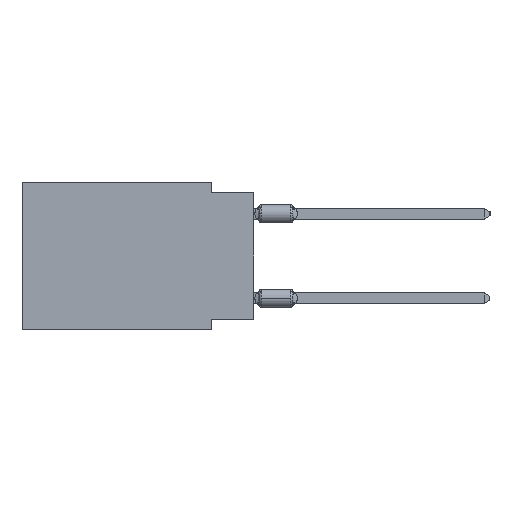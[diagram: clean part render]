
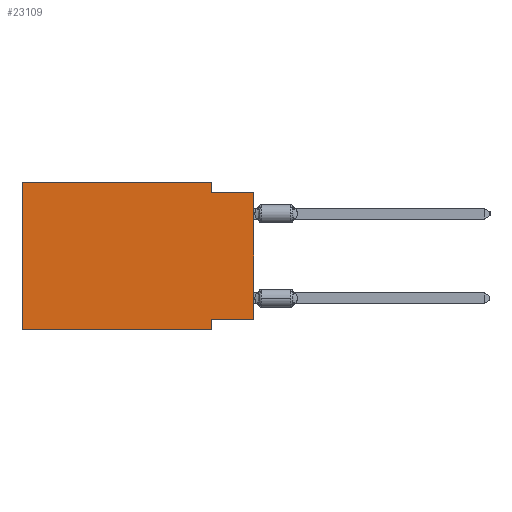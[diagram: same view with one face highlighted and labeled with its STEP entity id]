
A CAD part, left-side view. The second image highlights one B-rep face of the part: STEP entity #23109.
In plain terms, the highlighted planar face has unit normal (-1, 0, 0).
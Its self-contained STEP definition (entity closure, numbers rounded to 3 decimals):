
#933 = DIRECTION ( 'NONE',  ( 0., 1., 0. ) ) ;
#1464 = CARTESIAN_POINT ( 'NONE',  ( 0., 0., -8.255 ) ) ;
#4327 = VECTOR ( 'NONE', #4567, 1000. ) ;
#4567 = DIRECTION ( 'NONE',  ( 0., 0., -1. ) ) ;
#4967 = CARTESIAN_POINT ( 'NONE',  ( 0., 0., 0. ) ) ;
#5822 = ORIENTED_EDGE ( 'NONE', *, *, #59109, .F. ) ;
#6169 = FACE_OUTER_BOUND ( 'NONE', #55028, .T. ) ;
#6248 = CARTESIAN_POINT ( 'NONE',  ( 0., 13.97, 0. ) ) ;
#6306 = CARTESIAN_POINT ( 'NONE',  ( 0., 0., -8.255 ) ) ;
#6404 = EDGE_CURVE ( 'NONE', #53952, #66199, #46288, .T. ) ;
#6507 = PLANE ( 'NONE',  #38197 ) ;
#9650 = VECTOR ( 'NONE', #70091, 1000. ) ;
#11350 = LINE ( 'NONE', #65529, #69585 ) ;
#12468 = LINE ( 'NONE', #50595, #31604 ) ;
#14193 = ORIENTED_EDGE ( 'NONE', *, *, #14325, .T. ) ;
#14324 = EDGE_CURVE ( 'NONE', #34864, #66199, #17049, .T. ) ;
#14325 = EDGE_CURVE ( 'NONE', #20962, #28728, #11350, .T. ) ;
#17049 = LINE ( 'NONE', #4967, #24068 ) ;
#20962 = VERTEX_POINT ( 'NONE', #66958 ) ;
#22067 = DIRECTION ( 'NONE',  ( 0., 0., 1. ) ) ;
#22688 = CARTESIAN_POINT ( 'NONE',  ( 0., 2.54, -8.89 ) ) ;
#22704 = LINE ( 'NONE', #6306, #68304 ) ;
#23109 = ADVANCED_FACE ( 'NONE', ( #6169 ), #6507, .F. ) ;
#24068 = VECTOR ( 'NONE', #22067, 1000. ) ;
#25705 = EDGE_CURVE ( 'NONE', #61321, #30033, #12468, .T. ) ;
#26037 = CARTESIAN_POINT ( 'NONE',  ( 0., 2.54, -0.635 ) ) ;
#26087 = EDGE_CURVE ( 'NONE', #50773, #28728, #60484, .T. ) ;
#27874 = EDGE_CURVE ( 'NONE', #34864, #50773, #22704, .T. ) ;
#28728 = VERTEX_POINT ( 'NONE', #22688 ) ;
#29919 = CARTESIAN_POINT ( 'NONE',  ( 0., 0., -0.635 ) ) ;
#30033 = VERTEX_POINT ( 'NONE', #44791 ) ;
#30485 = EDGE_CURVE ( 'NONE', #30033, #53952, #37331, .T. ) ;
#31604 = VECTOR ( 'NONE', #60921, 1000. ) ;
#32894 = DIRECTION ( 'NONE',  ( 0., 0., -1. ) ) ;
#33108 = DIRECTION ( 'NONE',  ( 0., -1., 0. ) ) ;
#34864 = VERTEX_POINT ( 'NONE', #1464 ) ;
#37331 = LINE ( 'NONE', #59735, #9650 ) ;
#38197 = AXIS2_PLACEMENT_3D ( 'NONE', #44278, #49270, #32894 ) ;
#40005 = VECTOR ( 'NONE', #66470, 1000. ) ;
#44278 = CARTESIAN_POINT ( 'NONE',  ( 0., 13.97, 0. ) ) ;
#44791 = CARTESIAN_POINT ( 'NONE',  ( 0., 2.54, 0. ) ) ;
#46288 = LINE ( 'NONE', #29919, #47974 ) ;
#47299 = ORIENTED_EDGE ( 'NONE', *, *, #25705, .F. ) ;
#47974 = VECTOR ( 'NONE', #51631, 1000. ) ;
#48931 = ORIENTED_EDGE ( 'NONE', *, *, #30485, .F. ) ;
#49270 = DIRECTION ( 'NONE',  ( 1., 0., 0. ) ) ;
#49350 = LINE ( 'NONE', #6248, #40005 ) ;
#49409 = CARTESIAN_POINT ( 'NONE',  ( 0., 13.97, 0. ) ) ;
#50046 = ORIENTED_EDGE ( 'NONE', *, *, #14324, .T. ) ;
#50595 = CARTESIAN_POINT ( 'NONE',  ( 0., 13.97, 0. ) ) ;
#50773 = VERTEX_POINT ( 'NONE', #61368 ) ;
#51324 = ORIENTED_EDGE ( 'NONE', *, *, #6404, .F. ) ;
#51631 = DIRECTION ( 'NONE',  ( 0., -1., 0. ) ) ;
#53370 = CARTESIAN_POINT ( 'NONE',  ( 0., 2.54, -8.89 ) ) ;
#53952 = VERTEX_POINT ( 'NONE', #26037 ) ;
#55028 = EDGE_LOOP ( 'NONE', ( #50046, #51324, #48931, #47299, #5822, #14193, #58346, #61771 ) ) ;
#58346 = ORIENTED_EDGE ( 'NONE', *, *, #26087, .F. ) ;
#59109 = EDGE_CURVE ( 'NONE', #20962, #61321, #49350, .T. ) ;
#59735 = CARTESIAN_POINT ( 'NONE',  ( 0., 2.54, 0. ) ) ;
#60484 = LINE ( 'NONE', #53370, #4327 ) ;
#60921 = DIRECTION ( 'NONE',  ( 0., -1., 0. ) ) ;
#61321 = VERTEX_POINT ( 'NONE', #49409 ) ;
#61368 = CARTESIAN_POINT ( 'NONE',  ( 0., 2.54, -8.255 ) ) ;
#61771 = ORIENTED_EDGE ( 'NONE', *, *, #27874, .F. ) ;
#65529 = CARTESIAN_POINT ( 'NONE',  ( 0., 13.97, -8.89 ) ) ;
#66199 = VERTEX_POINT ( 'NONE', #66884 ) ;
#66470 = DIRECTION ( 'NONE',  ( 0., 0., 1. ) ) ;
#66884 = CARTESIAN_POINT ( 'NONE',  ( 0., 0., -0.635 ) ) ;
#66958 = CARTESIAN_POINT ( 'NONE',  ( 0., 13.97, -8.89 ) ) ;
#68304 = VECTOR ( 'NONE', #933, 1000. ) ;
#69585 = VECTOR ( 'NONE', #33108, 1000. ) ;
#70091 = DIRECTION ( 'NONE',  ( 0., 0., -1. ) ) ;
